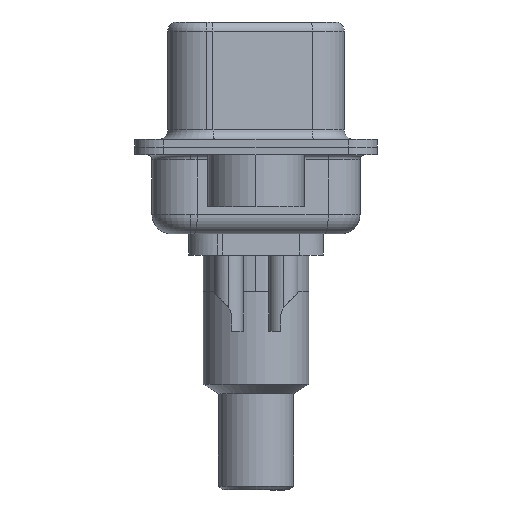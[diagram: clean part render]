
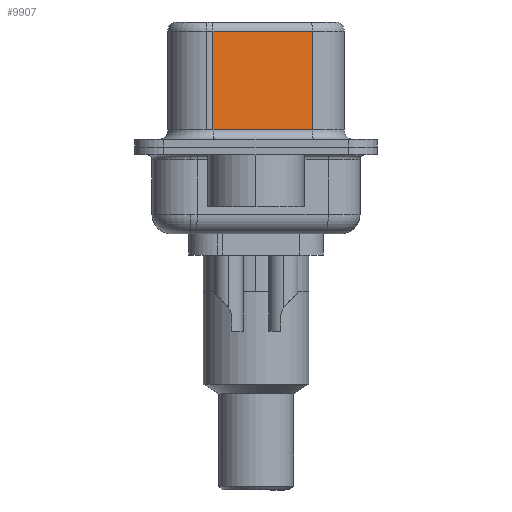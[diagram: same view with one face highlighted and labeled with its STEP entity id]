
A CAD part, left-side view. The second image highlights one B-rep face of the part: STEP entity #9907.
In plain terms, the highlighted planar face has unit normal (-0.985, -0.174, 0).
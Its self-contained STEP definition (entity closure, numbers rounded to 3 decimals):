
#745 = DIRECTION ( 'NONE',  ( 0.174, -0.985, 0. ) ) ;
#1445 = CARTESIAN_POINT ( 'NONE',  ( 3.655, 2.233, 6.02 ) ) ;
#1475 = LINE ( 'NONE', #7963, #19940 ) ;
#1513 = ORIENTED_EDGE ( 'NONE', *, *, #19829, .T. ) ;
#1785 = CARTESIAN_POINT ( 'NONE',  ( 4.565, -2.927, 6.52 ) ) ;
#2147 = FACE_OUTER_BOUND ( 'NONE', #9980, .T. ) ;
#2540 = VERTEX_POINT ( 'NONE', #6141 ) ;
#3538 = VERTEX_POINT ( 'NONE', #6756 ) ;
#4167 = VECTOR ( 'NONE', #18978, 1000. ) ;
#4374 = VECTOR ( 'NONE', #6210, 1000. ) ;
#5851 = VERTEX_POINT ( 'NONE', #13459 ) ;
#6141 = CARTESIAN_POINT ( 'NONE',  ( 4.565, -2.927, 6.02 ) ) ;
#6210 = DIRECTION ( 'NONE',  ( 0., 0., -1. ) ) ;
#6398 = CARTESIAN_POINT ( 'NONE',  ( 4.565, -2.927, 6.52 ) ) ;
#6665 = VERTEX_POINT ( 'NONE', #1445 ) ;
#6756 = CARTESIAN_POINT ( 'NONE',  ( 4.565, -2.927, 0.9 ) ) ;
#7963 = CARTESIAN_POINT ( 'NONE',  ( 4.565, -2.927, 0.9 ) ) ;
#8012 = VECTOR ( 'NONE', #15246, 1000. ) ;
#8396 = CARTESIAN_POINT ( 'NONE',  ( 4.565, -2.927, 6.02 ) ) ;
#9124 = PLANE ( 'NONE',  #11643 ) ;
#9907 = ADVANCED_FACE ( 'NONE', ( #2147 ), #9124, .F. ) ;
#9980 = EDGE_LOOP ( 'NONE', ( #16365, #1513, #22951, #19212 ) ) ;
#10896 = DIRECTION ( 'NONE',  ( -0.174, 0.985, 0. ) ) ;
#11643 = AXIS2_PLACEMENT_3D ( 'NONE', #1785, #21458, #10896 ) ;
#13459 = CARTESIAN_POINT ( 'NONE',  ( 3.655, 2.233, 0.9 ) ) ;
#14144 = LINE ( 'NONE', #8396, #4167 ) ;
#15246 = DIRECTION ( 'NONE',  ( 0., 0., -1. ) ) ;
#16365 = ORIENTED_EDGE ( 'NONE', *, *, #20854, .F. ) ;
#18507 = EDGE_CURVE ( 'NONE', #5851, #3538, #1475, .T. ) ;
#18591 = CARTESIAN_POINT ( 'NONE',  ( 3.655, 2.233, 6.52 ) ) ;
#18978 = DIRECTION ( 'NONE',  ( -0.174, 0.985, 0. ) ) ;
#19212 = ORIENTED_EDGE ( 'NONE', *, *, #18507, .T. ) ;
#19829 = EDGE_CURVE ( 'NONE', #2540, #6665, #14144, .T. ) ;
#19940 = VECTOR ( 'NONE', #745, 1000. ) ;
#20854 = EDGE_CURVE ( 'NONE', #2540, #3538, #21523, .T. ) ;
#21458 = DIRECTION ( 'NONE',  ( 0.985, 0.174, 0. ) ) ;
#21523 = LINE ( 'NONE', #6398, #8012 ) ;
#22055 = EDGE_CURVE ( 'NONE', #6665, #5851, #22614, .T. ) ;
#22614 = LINE ( 'NONE', #18591, #4374 ) ;
#22951 = ORIENTED_EDGE ( 'NONE', *, *, #22055, .T. ) ;
